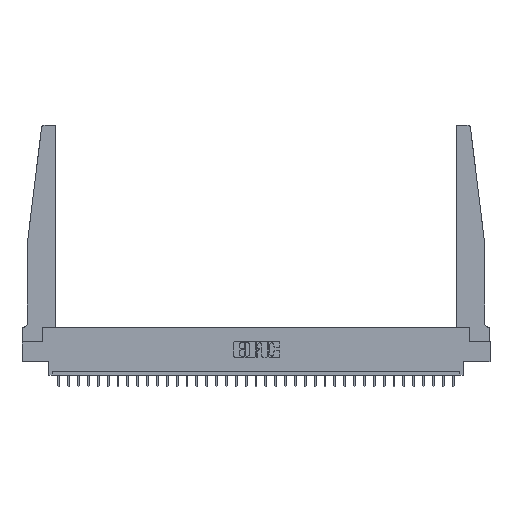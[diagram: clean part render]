
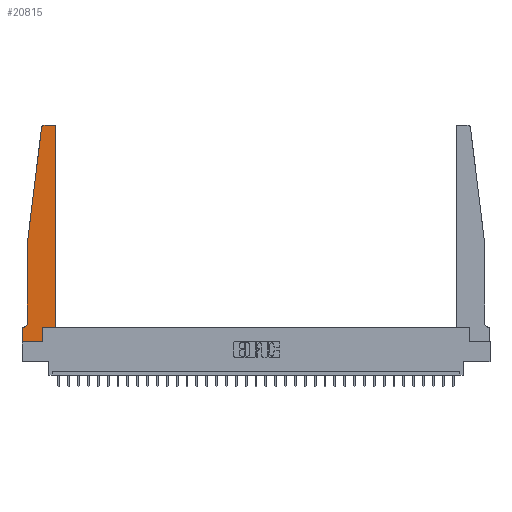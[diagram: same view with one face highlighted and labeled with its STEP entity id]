
A CAD part, top view. The second image highlights one B-rep face of the part: STEP entity #20815.
In plain terms, the highlighted planar face has unit normal (0, 0, 1).
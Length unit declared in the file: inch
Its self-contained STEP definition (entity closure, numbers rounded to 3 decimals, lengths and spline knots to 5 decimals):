
#414 = EDGE_CURVE ( 'NONE', #9595, #2075, #27694, .T. ) ;
#727 = DIRECTION ( 'NONE',  ( -0.122, -0.992, 0. ) ) ;
#778 = VERTEX_POINT ( 'NONE', #24543 ) ;
#919 = CARTESIAN_POINT ( 'NONE',  ( 0.2605, 0.18, 0.37 ) ) ;
#1027 = CARTESIAN_POINT ( 'NONE',  ( 0.425, 0.18, 0.37 ) ) ;
#1151 = EDGE_CURVE ( 'NONE', #23130, #778, #12240, .T. ) ;
#1333 = ORIENTED_EDGE ( 'NONE', *, *, #27110, .T. ) ;
#1945 = EDGE_CURVE ( 'NONE', #2075, #12465, #3329, .T. ) ;
#2075 = VERTEX_POINT ( 'NONE', #3444 ) ;
#2338 = VERTEX_POINT ( 'NONE', #919 ) ;
#2615 = DIRECTION ( 'NONE',  ( 0., 0., 1. ) ) ;
#2799 = VERTEX_POINT ( 'NONE', #25358 ) ;
#2804 = DIRECTION ( 'NONE',  ( 0., 1., 0. ) ) ;
#2837 = LINE ( 'NONE', #18055, #19871 ) ;
#3119 = VERTEX_POINT ( 'NONE', #22112 ) ;
#3156 = VECTOR ( 'NONE', #4847, 39.37008 ) ;
#3329 = CIRCLE ( 'NONE', #27797, 0.03 ) ;
#3432 = EDGE_CURVE ( 'NONE', #12465, #19064, #27919, .T. ) ;
#3444 = CARTESIAN_POINT ( 'NONE',  ( 0.425, 2.72, 0.37 ) ) ;
#3665 = ORIENTED_EDGE ( 'NONE', *, *, #414, .T. ) ;
#3722 = DIRECTION ( 'NONE',  ( 1., 0., 0. ) ) ;
#4126 = EDGE_CURVE ( 'NONE', #3119, #22397, #20483, .T. ) ;
#4603 = DIRECTION ( 'NONE',  ( 0., 0., 1. ) ) ;
#4847 = DIRECTION ( 'NONE',  ( 1., 0., 0. ) ) ;
#5134 = CARTESIAN_POINT ( 'NONE',  ( 0.425, 0.18, 0.37 ) ) ;
#5187 = ORIENTED_EDGE ( 'NONE', *, *, #11512, .T. ) ;
#5263 = DIRECTION ( 'NONE',  ( -1., 0., 0. ) ) ;
#5748 = LINE ( 'NONE', #1027, #27822 ) ;
#6640 = CARTESIAN_POINT ( 'NONE',  ( 0., 0., 0.37 ) ) ;
#6661 = CARTESIAN_POINT ( 'NONE',  ( 0.25, 2.75, 0.37 ) ) ;
#6826 = CARTESIAN_POINT ( 'NONE',  ( 0., 0.1875, 0.37 ) ) ;
#6995 = LINE ( 'NONE', #13963, #12520 ) ;
#7288 = CARTESIAN_POINT ( 'NONE',  ( 0.065, 0.2375, 0.37 ) ) ;
#7354 = CARTESIAN_POINT ( 'NONE',  ( 0.395, 2.72, 0.37 ) ) ;
#7647 = AXIS2_PLACEMENT_3D ( 'NONE', #16442, #19195, #16931 ) ;
#8242 = CIRCLE ( 'NONE', #7647, 0.05 ) ;
#8302 = LINE ( 'NONE', #25943, #3156 ) ;
#8752 = EDGE_CURVE ( 'NONE', #2799, #2338, #2837, .T. ) ;
#8885 = PLANE ( 'NONE',  #11822 ) ;
#9164 = VECTOR ( 'NONE', #5263, 39.37008 ) ;
#9595 = VERTEX_POINT ( 'NONE', #23899 ) ;
#10168 = DIRECTION ( 'NONE',  ( 1., 0., 0. ) ) ;
#10767 = VECTOR ( 'NONE', #727, 39.37008 ) ;
#10970 = DIRECTION ( 'NONE',  ( 0., -1., 0. ) ) ;
#11256 = ORIENTED_EDGE ( 'NONE', *, *, #3432, .T. ) ;
#11278 = CARTESIAN_POINT ( 'NONE',  ( 0., 0.1875, 0.37 ) ) ;
#11512 = EDGE_CURVE ( 'NONE', #22397, #30437, #6995, .T. ) ;
#11822 = AXIS2_PLACEMENT_3D ( 'NONE', #11278, #13637, #30087 ) ;
#11930 = CARTESIAN_POINT ( 'NONE',  ( 0.065, 1.25, 0.37 ) ) ;
#12240 = LINE ( 'NONE', #28823, #10767 ) ;
#12465 = VERTEX_POINT ( 'NONE', #22074 ) ;
#12520 = VECTOR ( 'NONE', #10970, 39.37008 ) ;
#13592 = ORIENTED_EDGE ( 'NONE', *, *, #21343, .T. ) ;
#13637 = DIRECTION ( 'NONE',  ( 0., 0., 1. ) ) ;
#13868 = ORIENTED_EDGE ( 'NONE', *, *, #19246, .T. ) ;
#13963 = CARTESIAN_POINT ( 'NONE',  ( 0., 0., 0.37 ) ) ;
#14105 = DIRECTION ( 'NONE',  ( 1., 0., 0. ) ) ;
#14187 = EDGE_LOOP ( 'NONE', ( #11256, #25812, #21510, #14356, #13592, #19341, #5187, #1333, #14449, #13868, #3665, #19966 ) ) ;
#14356 = ORIENTED_EDGE ( 'NONE', *, *, #24145, .T. ) ;
#14426 = CARTESIAN_POINT ( 'NONE',  ( 0.27653, 2.72, 0.37 ) ) ;
#14449 = ORIENTED_EDGE ( 'NONE', *, *, #8752, .T. ) ;
#14557 = VECTOR ( 'NONE', #17600, 39.37008 ) ;
#16442 = CARTESIAN_POINT ( 'NONE',  ( 0.015, 0.2375, 0.37 ) ) ;
#16504 = DIRECTION ( 'NONE',  ( 0., -1., 0. ) ) ;
#16931 = DIRECTION ( 'NONE',  ( -1., 0., 0. ) ) ;
#17154 = CIRCLE ( 'NONE', #27771, 0.03 ) ;
#17600 = DIRECTION ( 'NONE',  ( -1., 0., 0. ) ) ;
#17928 = CARTESIAN_POINT ( 'NONE',  ( 0.065, 0.1875, 0.37 ) ) ;
#18055 = CARTESIAN_POINT ( 'NONE',  ( 0.2605, 0.18, 0.37 ) ) ;
#18677 = CARTESIAN_POINT ( 'NONE',  ( 0.27653, 2.75, 0.37 ) ) ;
#19064 = VERTEX_POINT ( 'NONE', #18677 ) ;
#19182 = VECTOR ( 'NONE', #16504, 39.37008 ) ;
#19195 = DIRECTION ( 'NONE',  ( 0., 0., -1. ) ) ;
#19246 = EDGE_CURVE ( 'NONE', #2338, #9595, #5748, .T. ) ;
#19341 = ORIENTED_EDGE ( 'NONE', *, *, #4126, .T. ) ;
#19871 = VECTOR ( 'NONE', #2804, 39.37008 ) ;
#19966 = ORIENTED_EDGE ( 'NONE', *, *, #1945, .T. ) ;
#20483 = LINE ( 'NONE', #17928, #14557 ) ;
#20815 = ADVANCED_FACE ( 'NONE', ( #29976 ), #8885, .T. ) ;
#21343 = EDGE_CURVE ( 'NONE', #22026, #3119, #8242, .T. ) ;
#21510 = ORIENTED_EDGE ( 'NONE', *, *, #1151, .T. ) ;
#22026 = VERTEX_POINT ( 'NONE', #7288 ) ;
#22074 = CARTESIAN_POINT ( 'NONE',  ( 0.395, 2.75, 0.37 ) ) ;
#22112 = CARTESIAN_POINT ( 'NONE',  ( 0.015, 0.1875, 0.37 ) ) ;
#22397 = VERTEX_POINT ( 'NONE', #6826 ) ;
#23042 = CARTESIAN_POINT ( 'NONE',  ( 0.24675, 2.72367, 0.37 ) ) ;
#23130 = VERTEX_POINT ( 'NONE', #23042 ) ;
#23899 = CARTESIAN_POINT ( 'NONE',  ( 0.425, 0.18, 0.37 ) ) ;
#24145 = EDGE_CURVE ( 'NONE', #778, #22026, #25401, .T. ) ;
#24543 = CARTESIAN_POINT ( 'NONE',  ( 0.065, 1.25, 0.37 ) ) ;
#25358 = CARTESIAN_POINT ( 'NONE',  ( 0.2605, 0., 0.37 ) ) ;
#25401 = LINE ( 'NONE', #11930, #19182 ) ;
#25812 = ORIENTED_EDGE ( 'NONE', *, *, #27866, .T. ) ;
#25848 = DIRECTION ( 'NONE',  ( 0., 1., 0. ) ) ;
#25943 = CARTESIAN_POINT ( 'NONE',  ( 0., 0., 0.37 ) ) ;
#27110 = EDGE_CURVE ( 'NONE', #30437, #2799, #8302, .T. ) ;
#27318 = VECTOR ( 'NONE', #25848, 39.37008 ) ;
#27694 = LINE ( 'NONE', #5134, #27318 ) ;
#27771 = AXIS2_PLACEMENT_3D ( 'NONE', #14426, #2615, #10168 ) ;
#27797 = AXIS2_PLACEMENT_3D ( 'NONE', #7354, #4603, #14105 ) ;
#27822 = VECTOR ( 'NONE', #3722, 39.37008 ) ;
#27866 = EDGE_CURVE ( 'NONE', #19064, #23130, #17154, .T. ) ;
#27919 = LINE ( 'NONE', #6661, #9164 ) ;
#28823 = CARTESIAN_POINT ( 'NONE',  ( 0.065, 1.25, 0.37 ) ) ;
#29976 = FACE_OUTER_BOUND ( 'NONE', #14187, .T. ) ;
#30087 = DIRECTION ( 'NONE',  ( 1., 0., 0. ) ) ;
#30437 = VERTEX_POINT ( 'NONE', #6640 ) ;
